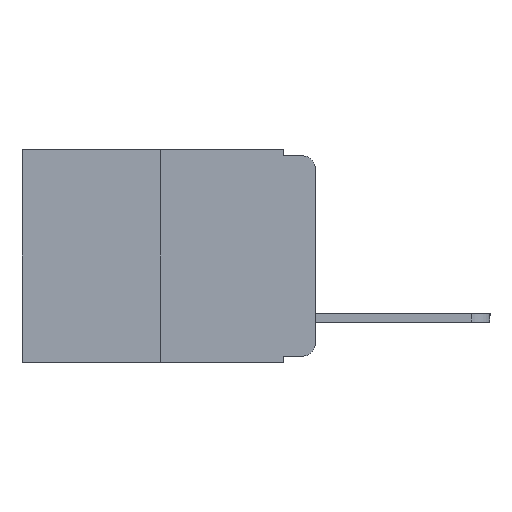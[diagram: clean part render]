
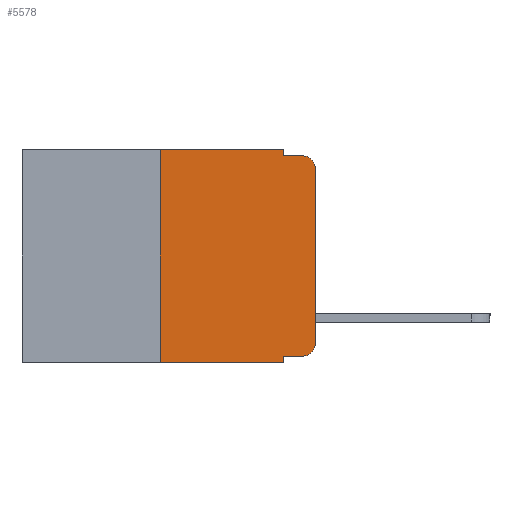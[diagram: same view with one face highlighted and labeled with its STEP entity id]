
A CAD part, left-side view. The second image highlights one B-rep face of the part: STEP entity #5578.
In plain terms, the highlighted planar face has unit normal (-1, 0, 0).
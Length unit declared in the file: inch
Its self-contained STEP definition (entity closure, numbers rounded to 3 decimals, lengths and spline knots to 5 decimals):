
#272 = CARTESIAN_POINT ( 'NONE',  ( 0., 0., 0. ) ) ;
#345 = CARTESIAN_POINT ( 'NONE',  ( 0., 0.473, -0.343 ) ) ;
#745 = VERTEX_POINT ( 'NONE', #1288 ) ;
#955 = DIRECTION ( 'NONE',  ( 0., 0., -1. ) ) ;
#965 = ORIENTED_EDGE ( 'NONE', *, *, #6730, .F. ) ;
#1027 = VERTEX_POINT ( 'NONE', #10568 ) ;
#1033 = LINE ( 'NONE', #6267, #1375 ) ;
#1246 = DIRECTION ( 'NONE',  ( -1., 0., 0. ) ) ;
#1288 = CARTESIAN_POINT ( 'NONE',  ( 0., 0.25, 0. ) ) ;
#1375 = VECTOR ( 'NONE', #955, 39.37008 ) ;
#1422 = CARTESIAN_POINT ( 'NONE',  ( 0., 0.051, -0.333 ) ) ;
#1539 = CIRCLE ( 'NONE', #10252, 0.02 ) ;
#1742 = LINE ( 'NONE', #345, #4273 ) ;
#2186 = CARTESIAN_POINT ( 'NONE',  ( 0., 0.051, -0.333 ) ) ;
#2332 = VERTEX_POINT ( 'NONE', #4885 ) ;
#2538 = PLANE ( 'NONE',  #5659 ) ;
#2602 = VERTEX_POINT ( 'NONE', #12323 ) ;
#2690 = CARTESIAN_POINT ( 'NONE',  ( 0., 0.473, 0. ) ) ;
#2782 = DIRECTION ( 'NONE',  ( 0., 0., 1. ) ) ;
#2845 = DIRECTION ( 'NONE',  ( -1., 0., 0. ) ) ;
#2946 = VERTEX_POINT ( 'NONE', #6650 ) ;
#3321 = VERTEX_POINT ( 'NONE', #3330 ) ;
#3330 = CARTESIAN_POINT ( 'NONE',  ( 0., 0., -0.03 ) ) ;
#3756 = EDGE_CURVE ( 'NONE', #745, #7491, #5448, .T. ) ;
#3842 = CARTESIAN_POINT ( 'NONE',  ( 0., 0.02, -0.01 ) ) ;
#3939 = VECTOR ( 'NONE', #7664, 39.37008 ) ;
#4098 = LINE ( 'NONE', #10536, #8919 ) ;
#4273 = VECTOR ( 'NONE', #11997, 39.37008 ) ;
#4717 = CARTESIAN_POINT ( 'NONE',  ( 0., 0.473, 0. ) ) ;
#4762 = VECTOR ( 'NONE', #10094, 39.37008 ) ;
#4806 = VERTEX_POINT ( 'NONE', #1422 ) ;
#4870 = ORIENTED_EDGE ( 'NONE', *, *, #7054, .F. ) ;
#4885 = CARTESIAN_POINT ( 'NONE',  ( 0., 0.25, -0.343 ) ) ;
#5014 = ORIENTED_EDGE ( 'NONE', *, *, #6472, .T. ) ;
#5248 = VECTOR ( 'NONE', #10229, 39.37008 ) ;
#5330 = VERTEX_POINT ( 'NONE', #8222 ) ;
#5448 = LINE ( 'NONE', #2690, #8038 ) ;
#5499 = ORIENTED_EDGE ( 'NONE', *, *, #7200, .F. ) ;
#5543 = LINE ( 'NONE', #272, #5248 ) ;
#5578 = ADVANCED_FACE ( 'NONE', ( #11675 ), #2538, .F. ) ;
#5659 = AXIS2_PLACEMENT_3D ( 'NONE', #4717, #11212, #5743 ) ;
#5743 = DIRECTION ( 'NONE',  ( 0., 0., -1. ) ) ;
#5814 = CARTESIAN_POINT ( 'NONE',  ( 0., 0.051, 0. ) ) ;
#5842 = ORIENTED_EDGE ( 'NONE', *, *, #7295, .T. ) ;
#6267 = CARTESIAN_POINT ( 'NONE',  ( 0., 0.051, 0. ) ) ;
#6305 = EDGE_CURVE ( 'NONE', #2602, #3321, #5543, .T. ) ;
#6472 = EDGE_CURVE ( 'NONE', #3321, #6489, #11940, .T. ) ;
#6489 = VERTEX_POINT ( 'NONE', #3842 ) ;
#6650 = CARTESIAN_POINT ( 'NONE',  ( 0., 0.051, -0.01 ) ) ;
#6730 = EDGE_CURVE ( 'NONE', #2946, #6489, #9506, .T. ) ;
#6893 = EDGE_CURVE ( 'NONE', #7491, #2946, #9066, .T. ) ;
#6900 = EDGE_CURVE ( 'NONE', #2332, #5330, #1742, .T. ) ;
#7054 = EDGE_CURVE ( 'NONE', #2332, #745, #4098, .T. ) ;
#7100 = AXIS2_PLACEMENT_3D ( 'NONE', #8752, #2845, #9668 ) ;
#7200 = EDGE_CURVE ( 'NONE', #4806, #5330, #1033, .T. ) ;
#7215 = ORIENTED_EDGE ( 'NONE', *, *, #3756, .F. ) ;
#7295 = EDGE_CURVE ( 'NONE', #4806, #1027, #7422, .T. ) ;
#7335 = EDGE_CURVE ( 'NONE', #1027, #2602, #1539, .T. ) ;
#7422 = LINE ( 'NONE', #2186, #4762 ) ;
#7491 = VERTEX_POINT ( 'NONE', #5814 ) ;
#7492 = CARTESIAN_POINT ( 'NONE',  ( 0., 0.02, -0.313 ) ) ;
#7664 = DIRECTION ( 'NONE',  ( 0., 0., -1. ) ) ;
#7792 = DIRECTION ( 'NONE',  ( 0., -1., 0. ) ) ;
#8038 = VECTOR ( 'NONE', #7792, 39.37008 ) ;
#8222 = CARTESIAN_POINT ( 'NONE',  ( 0., 0.051, -0.343 ) ) ;
#8335 = ORIENTED_EDGE ( 'NONE', *, *, #6900, .T. ) ;
#8372 = DIRECTION ( 'NONE',  ( 0., 0., -1. ) ) ;
#8484 = CARTESIAN_POINT ( 'NONE',  ( 0., 0.051, 0. ) ) ;
#8752 = CARTESIAN_POINT ( 'NONE',  ( 0., 0.02, -0.03 ) ) ;
#8919 = VECTOR ( 'NONE', #2782, 39.37008 ) ;
#9008 = ORIENTED_EDGE ( 'NONE', *, *, #6893, .F. ) ;
#9066 = LINE ( 'NONE', #8484, #3939 ) ;
#9069 = CARTESIAN_POINT ( 'NONE',  ( 0., 0.051, -0.01 ) ) ;
#9137 = ORIENTED_EDGE ( 'NONE', *, *, #6305, .T. ) ;
#9215 = VECTOR ( 'NONE', #9990, 39.37008 ) ;
#9506 = LINE ( 'NONE', #9069, #9215 ) ;
#9668 = DIRECTION ( 'NONE',  ( 0., 0., -1. ) ) ;
#9731 = ORIENTED_EDGE ( 'NONE', *, *, #7335, .T. ) ;
#9990 = DIRECTION ( 'NONE',  ( 0., -1., 0. ) ) ;
#10094 = DIRECTION ( 'NONE',  ( 0., -1., 0. ) ) ;
#10229 = DIRECTION ( 'NONE',  ( 0., 0., 1. ) ) ;
#10252 = AXIS2_PLACEMENT_3D ( 'NONE', #7492, #1246, #8372 ) ;
#10536 = CARTESIAN_POINT ( 'NONE',  ( 0., 0.25, 0. ) ) ;
#10568 = CARTESIAN_POINT ( 'NONE',  ( 0., 0.02, -0.333 ) ) ;
#11212 = DIRECTION ( 'NONE',  ( 1., 0., 0. ) ) ;
#11675 = FACE_OUTER_BOUND ( 'NONE', #12043, .T. ) ;
#11940 = CIRCLE ( 'NONE', #7100, 0.02 ) ;
#11997 = DIRECTION ( 'NONE',  ( 0., -1., 0. ) ) ;
#12043 = EDGE_LOOP ( 'NONE', ( #9137, #5014, #965, #9008, #7215, #4870, #8335, #5499, #5842, #9731 ) ) ;
#12323 = CARTESIAN_POINT ( 'NONE',  ( 0., 0., -0.313 ) ) ;
